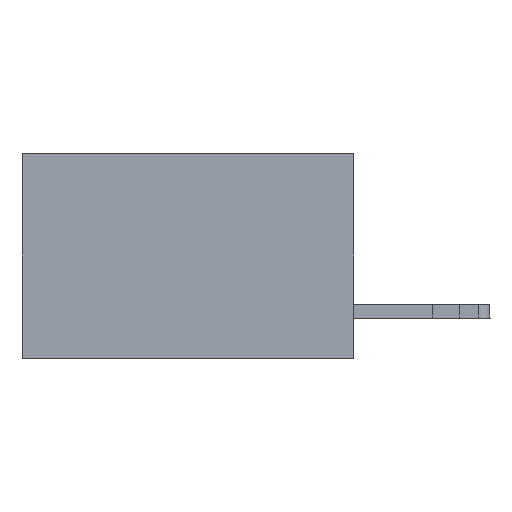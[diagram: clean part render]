
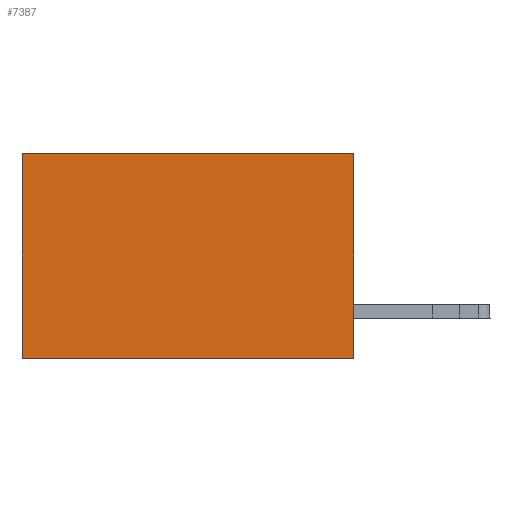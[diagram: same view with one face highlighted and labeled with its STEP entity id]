
A CAD part, left-side view. The second image highlights one B-rep face of the part: STEP entity #7387.
In plain terms, the highlighted planar face has unit normal (-1, 0, 0).
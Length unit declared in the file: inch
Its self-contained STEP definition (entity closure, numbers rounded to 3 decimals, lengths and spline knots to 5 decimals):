
#1161 = CARTESIAN_POINT ( 'NONE',  ( 0.2875, 0., -0.37 ) ) ;
#2062 = VERTEX_POINT ( 'NONE', #1161 ) ;
#2574 = VECTOR ( 'NONE', #28598, 39.37008 ) ;
#3157 = DIRECTION ( 'NONE',  ( 1., 0., 0. ) ) ;
#5229 = CARTESIAN_POINT ( 'NONE',  ( 0.2875, 0.6, -0.37 ) ) ;
#6060 = FACE_OUTER_BOUND ( 'NONE', #30885, .T. ) ;
#7387 = ADVANCED_FACE ( 'NONE', ( #6060 ), #27977, .F. ) ;
#9477 = CARTESIAN_POINT ( 'NONE',  ( 0.2875, 0.6, 0. ) ) ;
#11722 = VECTOR ( 'NONE', #28123, 39.37008 ) ;
#13667 = CARTESIAN_POINT ( 'NONE',  ( 0.2875, 0., -0.37 ) ) ;
#14005 = ORIENTED_EDGE ( 'NONE', *, *, #26296, .T. ) ;
#15255 = VECTOR ( 'NONE', #32715, 39.37008 ) ;
#16780 = VERTEX_POINT ( 'NONE', #31497 ) ;
#17732 = LINE ( 'NONE', #13667, #15255 ) ;
#18646 = EDGE_CURVE ( 'NONE', #16780, #2062, #28033, .T. ) ;
#19283 = VERTEX_POINT ( 'NONE', #22454 ) ;
#20626 = VECTOR ( 'NONE', #36691, 39.37008 ) ;
#21362 = AXIS2_PLACEMENT_3D ( 'NONE', #21827, #3157, #25104 ) ;
#21827 = CARTESIAN_POINT ( 'NONE',  ( 0.2875, 0., 0. ) ) ;
#21878 = ORIENTED_EDGE ( 'NONE', *, *, #34234, .T. ) ;
#22454 = CARTESIAN_POINT ( 'NONE',  ( 0.2875, 0.6, 0. ) ) ;
#25104 = DIRECTION ( 'NONE',  ( 0., 0., -1. ) ) ;
#26296 = EDGE_CURVE ( 'NONE', #16780, #19283, #37459, .T. ) ;
#26499 = ORIENTED_EDGE ( 'NONE', *, *, #32237, .F. ) ;
#27909 = VERTEX_POINT ( 'NONE', #5229 ) ;
#27977 = PLANE ( 'NONE',  #21362 ) ;
#28033 = LINE ( 'NONE', #37298, #20626 ) ;
#28123 = DIRECTION ( 'NONE',  ( 0., 0., -1. ) ) ;
#28509 = LINE ( 'NONE', #9477, #11722 ) ;
#28598 = DIRECTION ( 'NONE',  ( 0., 1., 0. ) ) ;
#30885 = EDGE_LOOP ( 'NONE', ( #21878, #26499, #38328, #14005 ) ) ;
#31497 = CARTESIAN_POINT ( 'NONE',  ( 0.2875, 0., 0. ) ) ;
#32237 = EDGE_CURVE ( 'NONE', #2062, #27909, #17732, .T. ) ;
#32715 = DIRECTION ( 'NONE',  ( 0., 1., 0. ) ) ;
#34234 = EDGE_CURVE ( 'NONE', #19283, #27909, #28509, .T. ) ;
#34374 = CARTESIAN_POINT ( 'NONE',  ( 0.2875, 0., 0. ) ) ;
#36691 = DIRECTION ( 'NONE',  ( 0., 0., -1. ) ) ;
#37298 = CARTESIAN_POINT ( 'NONE',  ( 0.2875, 0., 0. ) ) ;
#37459 = LINE ( 'NONE', #34374, #2574 ) ;
#38328 = ORIENTED_EDGE ( 'NONE', *, *, #18646, .F. ) ;
